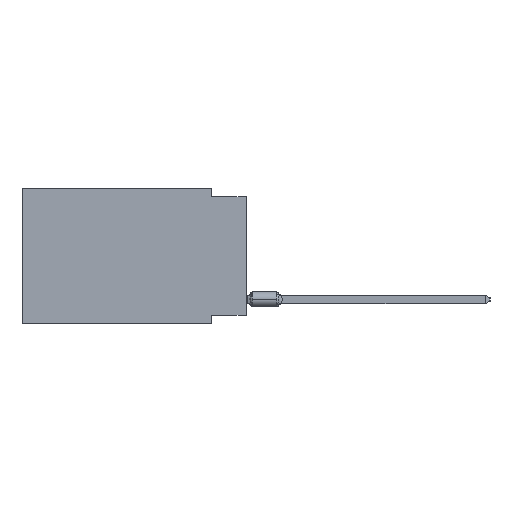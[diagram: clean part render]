
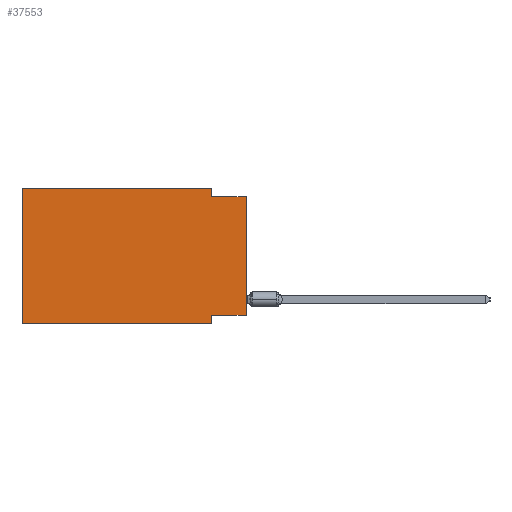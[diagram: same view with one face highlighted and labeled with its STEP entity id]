
A CAD part, left-side view. The second image highlights one B-rep face of the part: STEP entity #37553.
In plain terms, the highlighted planar face has unit normal (-1, 0, 0).
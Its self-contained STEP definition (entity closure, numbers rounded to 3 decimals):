
#586 = CARTESIAN_POINT ( 'NONE',  ( 0., 0., -0.635 ) ) ;
#1498 = LINE ( 'NONE', #79253, #15464 ) ;
#3701 = CARTESIAN_POINT ( 'NONE',  ( 0., 2.54, -9.906 ) ) ;
#4395 = VERTEX_POINT ( 'NONE', #586 ) ;
#5209 = VECTOR ( 'NONE', #38787, 1000. ) ;
#6964 = VERTEX_POINT ( 'NONE', #15454 ) ;
#7634 = ORIENTED_EDGE ( 'NONE', *, *, #72891, .F. ) ;
#7992 = CARTESIAN_POINT ( 'NONE',  ( 0., 2.54, 0. ) ) ;
#13227 = VECTOR ( 'NONE', #47005, 1000. ) ;
#14769 = ORIENTED_EDGE ( 'NONE', *, *, #27889, .F. ) ;
#15454 = CARTESIAN_POINT ( 'NONE',  ( 0., 2.54, -0.635 ) ) ;
#15464 = VECTOR ( 'NONE', #29519, 1000. ) ;
#15565 = ORIENTED_EDGE ( 'NONE', *, *, #58538, .F. ) ;
#17042 = LINE ( 'NONE', #43408, #66455 ) ;
#18328 = LINE ( 'NONE', #63803, #73932 ) ;
#18872 = CARTESIAN_POINT ( 'NONE',  ( 0., 16.383, 0. ) ) ;
#20242 = CARTESIAN_POINT ( 'NONE',  ( 0., 0., -9.271 ) ) ;
#20478 = CARTESIAN_POINT ( 'NONE',  ( 0., 2.54, -9.906 ) ) ;
#21776 = VECTOR ( 'NONE', #83286, 1000. ) ;
#22072 = CARTESIAN_POINT ( 'NONE',  ( 0., 16.383, -9.906 ) ) ;
#24522 = VERTEX_POINT ( 'NONE', #51523 ) ;
#24811 = LINE ( 'NONE', #18872, #45541 ) ;
#27361 = ORIENTED_EDGE ( 'NONE', *, *, #71761, .F. ) ;
#27889 = EDGE_CURVE ( 'NONE', #49872, #28366, #75495, .T. ) ;
#28108 = VERTEX_POINT ( 'NONE', #73728 ) ;
#28366 = VERTEX_POINT ( 'NONE', #70700 ) ;
#29519 = DIRECTION ( 'NONE',  ( 0., 0., 1. ) ) ;
#31219 = DIRECTION ( 'NONE',  ( 0., 0., -1. ) ) ;
#35824 = VERTEX_POINT ( 'NONE', #3701 ) ;
#37553 = ADVANCED_FACE ( 'NONE', ( #64337 ), #39671, .F. ) ;
#37894 = LINE ( 'NONE', #77783, #21776 ) ;
#38787 = DIRECTION ( 'NONE',  ( 0., 0., -1. ) ) ;
#39005 = EDGE_CURVE ( 'NONE', #64545, #6964, #37894, .T. ) ;
#39618 = LINE ( 'NONE', #20478, #5209 ) ;
#39671 = PLANE ( 'NONE',  #49024 ) ;
#40989 = ORIENTED_EDGE ( 'NONE', *, *, #66144, .T. ) ;
#41985 = ORIENTED_EDGE ( 'NONE', *, *, #39005, .F. ) ;
#42986 = DIRECTION ( 'NONE',  ( 0., -1., 0. ) ) ;
#43408 = CARTESIAN_POINT ( 'NONE',  ( 0., 16.383, -9.906 ) ) ;
#45541 = VECTOR ( 'NONE', #50759, 1000. ) ;
#46054 = DIRECTION ( 'NONE',  ( 1., 0., 0. ) ) ;
#47005 = DIRECTION ( 'NONE',  ( 0., 1., 0. ) ) ;
#47867 = VECTOR ( 'NONE', #75925, 1000. ) ;
#49024 = AXIS2_PLACEMENT_3D ( 'NONE', #76665, #46054, #31219 ) ;
#49872 = VERTEX_POINT ( 'NONE', #22072 ) ;
#50759 = DIRECTION ( 'NONE',  ( 0., -1., 0. ) ) ;
#51523 = CARTESIAN_POINT ( 'NONE',  ( 0., 0., -9.271 ) ) ;
#54756 = ORIENTED_EDGE ( 'NONE', *, *, #76225, .F. ) ;
#55426 = ORIENTED_EDGE ( 'NONE', *, *, #65047, .T. ) ;
#56366 = CARTESIAN_POINT ( 'NONE',  ( 0., 16.383, 0. ) ) ;
#58538 = EDGE_CURVE ( 'NONE', #28108, #35824, #39618, .T. ) ;
#58677 = DIRECTION ( 'NONE',  ( 0., -1., 0. ) ) ;
#63803 = CARTESIAN_POINT ( 'NONE',  ( 0., 0., -0.635 ) ) ;
#64337 = FACE_OUTER_BOUND ( 'NONE', #64820, .T. ) ;
#64545 = VERTEX_POINT ( 'NONE', #7992 ) ;
#64820 = EDGE_LOOP ( 'NONE', ( #55426, #27361, #41985, #7634, #14769, #40989, #15565, #54756 ) ) ;
#65047 = EDGE_CURVE ( 'NONE', #24522, #4395, #1498, .T. ) ;
#66144 = EDGE_CURVE ( 'NONE', #49872, #35824, #17042, .T. ) ;
#66455 = VECTOR ( 'NONE', #42986, 1000. ) ;
#66547 = LINE ( 'NONE', #20242, #13227 ) ;
#70700 = CARTESIAN_POINT ( 'NONE',  ( 0., 16.383, 0. ) ) ;
#71761 = EDGE_CURVE ( 'NONE', #6964, #4395, #18328, .T. ) ;
#72891 = EDGE_CURVE ( 'NONE', #28366, #64545, #24811, .T. ) ;
#73728 = CARTESIAN_POINT ( 'NONE',  ( 0., 2.54, -9.271 ) ) ;
#73932 = VECTOR ( 'NONE', #58677, 1000. ) ;
#75495 = LINE ( 'NONE', #56366, #47867 ) ;
#75925 = DIRECTION ( 'NONE',  ( 0., 0., 1. ) ) ;
#76225 = EDGE_CURVE ( 'NONE', #24522, #28108, #66547, .T. ) ;
#76665 = CARTESIAN_POINT ( 'NONE',  ( 0., 16.383, 0. ) ) ;
#77783 = CARTESIAN_POINT ( 'NONE',  ( 0., 2.54, 0. ) ) ;
#79253 = CARTESIAN_POINT ( 'NONE',  ( 0., 0., 0. ) ) ;
#83286 = DIRECTION ( 'NONE',  ( 0., 0., -1. ) ) ;
